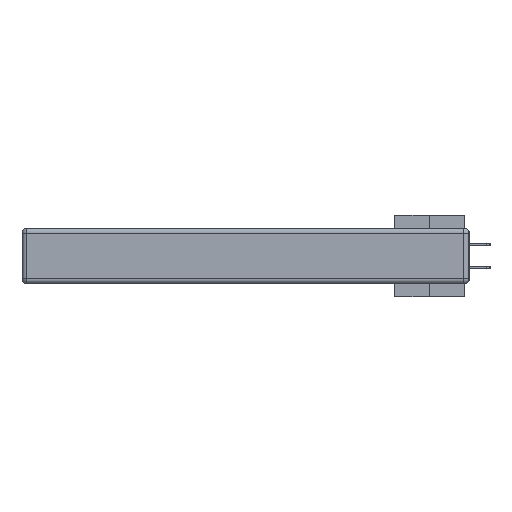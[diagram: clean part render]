
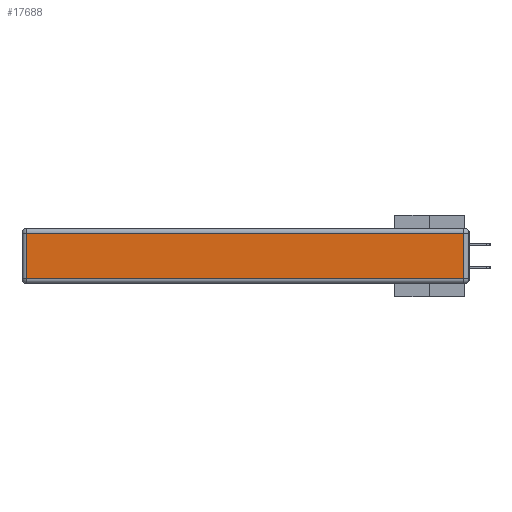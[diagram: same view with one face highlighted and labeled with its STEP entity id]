
A CAD part, left-side view. The second image highlights one B-rep face of the part: STEP entity #17688.
In plain terms, the highlighted planar face has unit normal (-1, 0, 0).
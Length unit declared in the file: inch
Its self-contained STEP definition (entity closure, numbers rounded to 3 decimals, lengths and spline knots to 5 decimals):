
#505 = VECTOR ( 'NONE', #15760, 39.37008 ) ;
#1658 = EDGE_CURVE ( 'NONE', #32614, #11425, #16823, .T. ) ;
#2434 = AXIS2_PLACEMENT_3D ( 'NONE', #24319, #24087, #19063 ) ;
#4501 = ORIENTED_EDGE ( 'NONE', *, *, #19318, .T. ) ;
#6281 = FACE_OUTER_BOUND ( 'NONE', #24953, .T. ) ;
#7804 = CARTESIAN_POINT ( 'NONE',  ( 0., 2.72, -0.03 ) ) ;
#9143 = CARTESIAN_POINT ( 'NONE',  ( 0., 2.72, -0.313 ) ) ;
#9227 = DIRECTION ( 'NONE',  ( 0., 0., 1. ) ) ;
#10198 = VERTEX_POINT ( 'NONE', #7804 ) ;
#10235 = VECTOR ( 'NONE', #15589, 39.37008 ) ;
#11313 = ORIENTED_EDGE ( 'NONE', *, *, #15825, .T. ) ;
#11425 = VERTEX_POINT ( 'NONE', #34534 ) ;
#13627 = ORIENTED_EDGE ( 'NONE', *, *, #26089, .T. ) ;
#14788 = CARTESIAN_POINT ( 'NONE',  ( 0., 0.03, -0.313 ) ) ;
#15589 = DIRECTION ( 'NONE',  ( 0., 1., 0. ) ) ;
#15687 = VECTOR ( 'NONE', #18163, 39.37008 ) ;
#15760 = DIRECTION ( 'NONE',  ( 0., -1., 0. ) ) ;
#15825 = EDGE_CURVE ( 'NONE', #11425, #10198, #20683, .T. ) ;
#16823 = LINE ( 'NONE', #25279, #17225 ) ;
#17225 = VECTOR ( 'NONE', #9227, 39.37008 ) ;
#17688 = ADVANCED_FACE ( 'NONE', ( #6281 ), #21411, .T. ) ;
#18163 = DIRECTION ( 'NONE',  ( 0., 0., -1. ) ) ;
#19063 = DIRECTION ( 'NONE',  ( 0., 0., 1. ) ) ;
#19318 = EDGE_CURVE ( 'NONE', #10198, #21877, #30309, .T. ) ;
#19686 = ORIENTED_EDGE ( 'NONE', *, *, #1658, .T. ) ;
#20641 = CARTESIAN_POINT ( 'NONE',  ( 0., 2.75, -0.03 ) ) ;
#20683 = LINE ( 'NONE', #20641, #10235 ) ;
#21411 = PLANE ( 'NONE',  #2434 ) ;
#21877 = VERTEX_POINT ( 'NONE', #9143 ) ;
#21909 = LINE ( 'NONE', #26102, #505 ) ;
#23289 = CARTESIAN_POINT ( 'NONE',  ( 0., 2.72, -0.343 ) ) ;
#24087 = DIRECTION ( 'NONE',  ( -1., 0., 0. ) ) ;
#24319 = CARTESIAN_POINT ( 'NONE',  ( 0., 0., -0.343 ) ) ;
#24953 = EDGE_LOOP ( 'NONE', ( #13627, #19686, #11313, #4501 ) ) ;
#25279 = CARTESIAN_POINT ( 'NONE',  ( 0., 0.03, -0.343 ) ) ;
#26089 = EDGE_CURVE ( 'NONE', #21877, #32614, #21909, .T. ) ;
#26102 = CARTESIAN_POINT ( 'NONE',  ( 0., 0., -0.313 ) ) ;
#30309 = LINE ( 'NONE', #23289, #15687 ) ;
#32614 = VERTEX_POINT ( 'NONE', #14788 ) ;
#34534 = CARTESIAN_POINT ( 'NONE',  ( 0., 0.03, -0.03 ) ) ;
